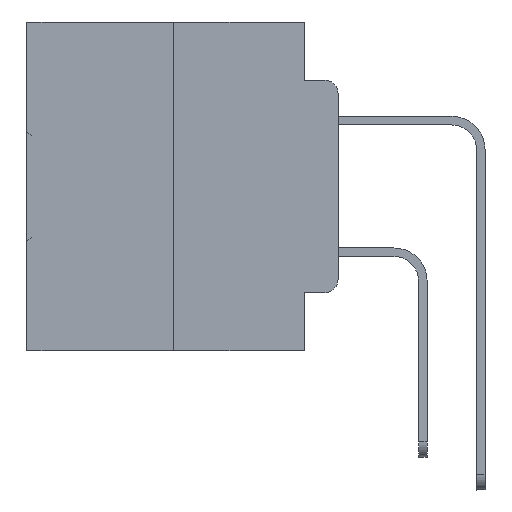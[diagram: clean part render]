
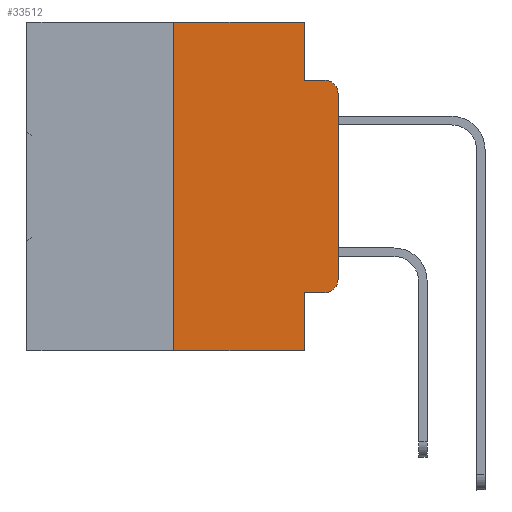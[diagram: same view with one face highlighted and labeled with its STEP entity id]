
A CAD part, left-side view. The second image highlights one B-rep face of the part: STEP entity #33512.
In plain terms, the highlighted planar face has unit normal (-1, 0, 0).
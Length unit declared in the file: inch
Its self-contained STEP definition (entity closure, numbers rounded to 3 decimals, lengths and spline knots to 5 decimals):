
#115 = CARTESIAN_POINT ( 'NONE',  ( 0., 0.473, 0. ) ) ;
#1107 = DIRECTION ( 'NONE',  ( 0., 0., -1. ) ) ;
#1199 = ORIENTED_EDGE ( 'NONE', *, *, #24013, .F. ) ;
#1513 = DIRECTION ( 'NONE',  ( 0., 0., 1. ) ) ;
#1795 = DIRECTION ( 'NONE',  ( 0., 0., -1. ) ) ;
#1874 = AXIS2_PLACEMENT_3D ( 'NONE', #7140, #4200, #32234 ) ;
#1954 = VECTOR ( 'NONE', #15973, 39.37008 ) ;
#2557 = ORIENTED_EDGE ( 'NONE', *, *, #21705, .T. ) ;
#3944 = CARTESIAN_POINT ( 'NONE',  ( 0., 0.02, -0.4115 ) ) ;
#4070 = EDGE_CURVE ( 'NONE', #24694, #22023, #26433, .T. ) ;
#4200 = DIRECTION ( 'NONE',  ( -1., 0., 0. ) ) ;
#4579 = DIRECTION ( 'NONE',  ( 0., 0., 1. ) ) ;
#4672 = DIRECTION ( 'NONE',  ( 0., -1., 0. ) ) ;
#6144 = CARTESIAN_POINT ( 'NONE',  ( 0., 0.051, -0.4115 ) ) ;
#6581 = AXIS2_PLACEMENT_3D ( 'NONE', #7104, #18267, #14989 ) ;
#6798 = LINE ( 'NONE', #20890, #15352 ) ;
#7104 = CARTESIAN_POINT ( 'NONE',  ( 0., 0.02, -0.3915 ) ) ;
#7140 = CARTESIAN_POINT ( 'NONE',  ( 0., 0.02, -0.1085 ) ) ;
#7217 = EDGE_CURVE ( 'NONE', #15370, #15635, #33474, .T. ) ;
#7565 = VERTEX_POINT ( 'NONE', #28544 ) ;
#9092 = ORIENTED_EDGE ( 'NONE', *, *, #21002, .T. ) ;
#10531 = LINE ( 'NONE', #27376, #19297 ) ;
#10834 = VECTOR ( 'NONE', #1107, 39.37008 ) ;
#11266 = EDGE_CURVE ( 'NONE', #26815, #15635, #16161, .T. ) ;
#11509 = CARTESIAN_POINT ( 'NONE',  ( 0., 0.02, -0.0885 ) ) ;
#11583 = DIRECTION ( 'NONE',  ( 0., -1., 0. ) ) ;
#11849 = DIRECTION ( 'NONE',  ( 1., 0., 0. ) ) ;
#12468 = EDGE_CURVE ( 'NONE', #32263, #7565, #15919, .T. ) ;
#13057 = CARTESIAN_POINT ( 'NONE',  ( 0., 0.051, -0.0885 ) ) ;
#13209 = VECTOR ( 'NONE', #11583, 39.37008 ) ;
#13644 = LINE ( 'NONE', #24809, #19638 ) ;
#14337 = ORIENTED_EDGE ( 'NONE', *, *, #4070, .F. ) ;
#14396 = FACE_OUTER_BOUND ( 'NONE', #20164, .T. ) ;
#14730 = CARTESIAN_POINT ( 'NONE',  ( 0., 0.25, -0.5 ) ) ;
#14738 = EDGE_CURVE ( 'NONE', #24694, #7565, #13644, .T. ) ;
#14989 = DIRECTION ( 'NONE',  ( 0., 0., -1. ) ) ;
#15247 = ORIENTED_EDGE ( 'NONE', *, *, #35684, .F. ) ;
#15352 = VECTOR ( 'NONE', #4579, 39.37008 ) ;
#15370 = VERTEX_POINT ( 'NONE', #28240 ) ;
#15397 = AXIS2_PLACEMENT_3D ( 'NONE', #115, #11849, #34188 ) ;
#15635 = VERTEX_POINT ( 'NONE', #11509 ) ;
#15919 = LINE ( 'NONE', #25084, #10834 ) ;
#15973 = DIRECTION ( 'NONE',  ( 0., -1., 0. ) ) ;
#16159 = VERTEX_POINT ( 'NONE', #3944 ) ;
#16161 = LINE ( 'NONE', #13057, #1954 ) ;
#17299 = VECTOR ( 'NONE', #1513, 39.37008 ) ;
#17678 = CIRCLE ( 'NONE', #6581, 0.02 ) ;
#18115 = LINE ( 'NONE', #18281, #19504 ) ;
#18267 = DIRECTION ( 'NONE',  ( -1., 0., 0. ) ) ;
#18281 = CARTESIAN_POINT ( 'NONE',  ( 0., 0.051, 0. ) ) ;
#18370 = VERTEX_POINT ( 'NONE', #26357 ) ;
#18933 = EDGE_CURVE ( 'NONE', #32263, #16159, #10531, .T. ) ;
#19036 = ORIENTED_EDGE ( 'NONE', *, *, #14738, .T. ) ;
#19297 = VECTOR ( 'NONE', #21676, 39.37008 ) ;
#19504 = VECTOR ( 'NONE', #1795, 39.37008 ) ;
#19638 = VECTOR ( 'NONE', #4672, 39.37008 ) ;
#19716 = PLANE ( 'NONE',  #15397 ) ;
#20164 = EDGE_LOOP ( 'NONE', ( #2557, #31677, #35879, #1199, #15247, #14337, #19036, #32003, #33197, #9092 ) ) ;
#20890 = CARTESIAN_POINT ( 'NONE',  ( 0., 0., 0. ) ) ;
#21002 = EDGE_CURVE ( 'NONE', #16159, #18370, #17678, .T. ) ;
#21676 = DIRECTION ( 'NONE',  ( 0., -1., 0. ) ) ;
#21705 = EDGE_CURVE ( 'NONE', #18370, #15370, #6798, .T. ) ;
#22023 = VERTEX_POINT ( 'NONE', #30961 ) ;
#22364 = LINE ( 'NONE', #30833, #13209 ) ;
#23486 = CARTESIAN_POINT ( 'NONE',  ( 0., 0.25, 0. ) ) ;
#24013 = EDGE_CURVE ( 'NONE', #28412, #26815, #18115, .T. ) ;
#24694 = VERTEX_POINT ( 'NONE', #14730 ) ;
#24809 = CARTESIAN_POINT ( 'NONE',  ( 0., 0.473, -0.5 ) ) ;
#25084 = CARTESIAN_POINT ( 'NONE',  ( 0., 0.051, 0. ) ) ;
#26003 = CARTESIAN_POINT ( 'NONE',  ( 0., 0.051, 0. ) ) ;
#26357 = CARTESIAN_POINT ( 'NONE',  ( 0., 0., -0.3915 ) ) ;
#26433 = LINE ( 'NONE', #23486, #17299 ) ;
#26815 = VERTEX_POINT ( 'NONE', #30607 ) ;
#27376 = CARTESIAN_POINT ( 'NONE',  ( 0., 0.051, -0.4115 ) ) ;
#28240 = CARTESIAN_POINT ( 'NONE',  ( 0., 0., -0.1085 ) ) ;
#28412 = VERTEX_POINT ( 'NONE', #26003 ) ;
#28544 = CARTESIAN_POINT ( 'NONE',  ( 0., 0.051, -0.5 ) ) ;
#30607 = CARTESIAN_POINT ( 'NONE',  ( 0., 0.051, -0.0885 ) ) ;
#30833 = CARTESIAN_POINT ( 'NONE',  ( 0., 0.473, 0. ) ) ;
#30961 = CARTESIAN_POINT ( 'NONE',  ( 0., 0.25, 0. ) ) ;
#31677 = ORIENTED_EDGE ( 'NONE', *, *, #7217, .T. ) ;
#32003 = ORIENTED_EDGE ( 'NONE', *, *, #12468, .F. ) ;
#32234 = DIRECTION ( 'NONE',  ( 0., 0., -1. ) ) ;
#32263 = VERTEX_POINT ( 'NONE', #6144 ) ;
#33197 = ORIENTED_EDGE ( 'NONE', *, *, #18933, .T. ) ;
#33474 = CIRCLE ( 'NONE', #1874, 0.02 ) ;
#33512 = ADVANCED_FACE ( 'NONE', ( #14396 ), #19716, .F. ) ;
#34188 = DIRECTION ( 'NONE',  ( 0., 0., -1. ) ) ;
#35684 = EDGE_CURVE ( 'NONE', #22023, #28412, #22364, .T. ) ;
#35879 = ORIENTED_EDGE ( 'NONE', *, *, #11266, .F. ) ;
